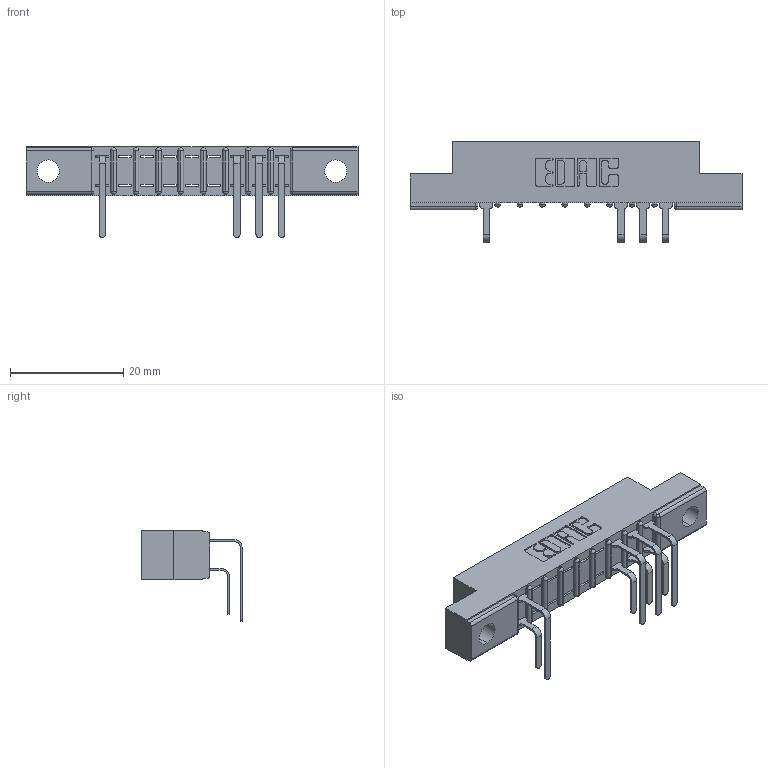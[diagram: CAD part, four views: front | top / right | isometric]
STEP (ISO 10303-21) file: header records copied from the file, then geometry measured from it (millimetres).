
FILE_DESCRIPTION (( 'STEP AP203' ), '1' );
FILE_NAME ('357-009-559-102.STEP', '2018-08-07T01:52:25', ( '' ), ( '' ), 'SwSTEP 2.0', 'SolidWorks 2016', '' );
FILE_SCHEMA (( 'CONFIG_CONTROL_DESIGN' ));
Length unit declared in the file: inch
Products named in the file (4): 307 Part_.128 Dia Mounting Holes; 307-290-001_558 559 - 1 (Single); 307-290-001_559 - 2 (Single); 357-009-559-102
Assembly tree (9 placements, depth 2):
  357-009-559-102
    307 Part_.128 Dia Mounting Holes
    307-290-001_558 559 - 1 (Single)  x4
    307-290-001_559 - 2 (Single)  x4
Bounding box: 58.67 x 17.69 x 16.08 mm (x, y, z)
Volume: 3657.5 mm3; surface area: 5064 mm2
Topology: 9 solids, 9 shells, 628 faces, 1779 edges, 1146 vertices
Faces by surface type: plane 394, cylinder 214, sphere 20
Entity records: 13201 total; most frequent: CARTESIAN_POINT 2213, ORIENTED_EDGE 2198, DIRECTION 2171, EDGE_CURVE 1099, LINE 827, VECTOR 827, VERTEX_POINT 714, AXIS2_PLACEMENT_3D 672
